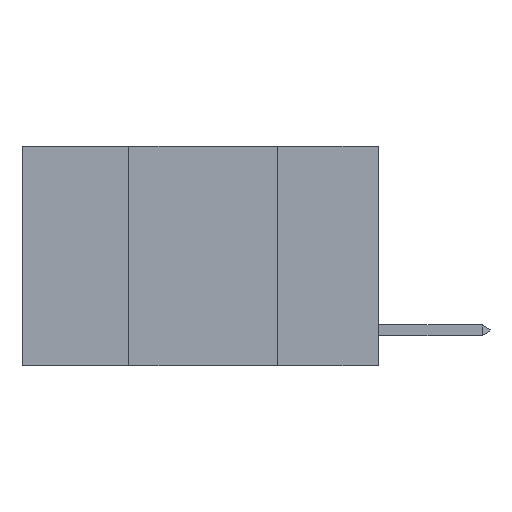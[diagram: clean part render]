
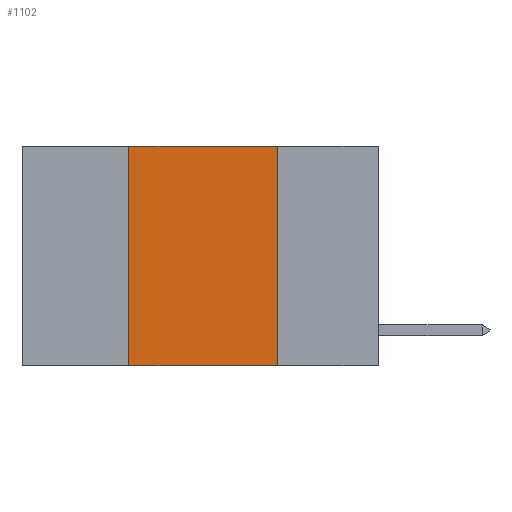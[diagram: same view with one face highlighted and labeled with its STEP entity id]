
A CAD part, left-side view. The second image highlights one B-rep face of the part: STEP entity #1102.
In plain terms, the highlighted planar face has unit normal (-1, 0, 0).
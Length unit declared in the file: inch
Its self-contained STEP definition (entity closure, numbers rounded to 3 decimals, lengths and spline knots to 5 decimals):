
#64 = CARTESIAN_POINT ( 'NONE',  ( 0., 0.6, -0.37 ) ) ;
#1066 = DIRECTION ( 'NONE',  ( 0., 0., 1. ) ) ;
#1102 = ADVANCED_FACE ( 'NONE', ( #3774 ), #3610, .F. ) ;
#1145 = LINE ( 'NONE', #4390, #6792 ) ;
#1159 = LINE ( 'NONE', #9218, #4058 ) ;
#1270 = DIRECTION ( 'NONE',  ( 0., 0., -1. ) ) ;
#1675 = VERTEX_POINT ( 'NONE', #3170 ) ;
#2013 = CARTESIAN_POINT ( 'NONE',  ( 0., 0.6, 0. ) ) ;
#2267 = EDGE_LOOP ( 'NONE', ( #5876, #2922, #2839, #2470 ) ) ;
#2470 = ORIENTED_EDGE ( 'NONE', *, *, #8190, .T. ) ;
#2485 = CARTESIAN_POINT ( 'NONE',  ( 0., 0.17, -0.37 ) ) ;
#2839 = ORIENTED_EDGE ( 'NONE', *, *, #3211, .F. ) ;
#2922 = ORIENTED_EDGE ( 'NONE', *, *, #9535, .F. ) ;
#3001 = AXIS2_PLACEMENT_3D ( 'NONE', #2013, #3715, #1270 ) ;
#3170 = CARTESIAN_POINT ( 'NONE',  ( 0., 0.17, 0. ) ) ;
#3211 = EDGE_CURVE ( 'NONE', #5841, #7922, #1159, .T. ) ;
#3424 = VERTEX_POINT ( 'NONE', #2485 ) ;
#3610 = PLANE ( 'NONE',  #3001 ) ;
#3715 = DIRECTION ( 'NONE',  ( 1., 0., 0. ) ) ;
#3774 = FACE_OUTER_BOUND ( 'NONE', #2267, .T. ) ;
#3865 = VECTOR ( 'NONE', #5063, 39.37008 ) ;
#4058 = VECTOR ( 'NONE', #1066, 39.37008 ) ;
#4250 = LINE ( 'NONE', #64, #3865 ) ;
#4363 = VECTOR ( 'NONE', #7636, 39.37008 ) ;
#4390 = CARTESIAN_POINT ( 'NONE',  ( 0., 0.17, 0. ) ) ;
#4437 = DIRECTION ( 'NONE',  ( 0., 0., -1. ) ) ;
#5063 = DIRECTION ( 'NONE',  ( 0., -1., 0. ) ) ;
#5147 = CARTESIAN_POINT ( 'NONE',  ( 0., 0.42, 0. ) ) ;
#5777 = CARTESIAN_POINT ( 'NONE',  ( 0., 0.42, -0.37 ) ) ;
#5841 = VERTEX_POINT ( 'NONE', #5777 ) ;
#5876 = ORIENTED_EDGE ( 'NONE', *, *, #7526, .F. ) ;
#6792 = VECTOR ( 'NONE', #4437, 39.37008 ) ;
#7526 = EDGE_CURVE ( 'NONE', #1675, #3424, #1145, .T. ) ;
#7636 = DIRECTION ( 'NONE',  ( 0., -1., 0. ) ) ;
#7922 = VERTEX_POINT ( 'NONE', #5147 ) ;
#8190 = EDGE_CURVE ( 'NONE', #5841, #3424, #4250, .T. ) ;
#9020 = CARTESIAN_POINT ( 'NONE',  ( 0., 0.6, 0. ) ) ;
#9127 = LINE ( 'NONE', #9020, #4363 ) ;
#9218 = CARTESIAN_POINT ( 'NONE',  ( 0., 0.42, 0. ) ) ;
#9535 = EDGE_CURVE ( 'NONE', #7922, #1675, #9127, .T. ) ;
